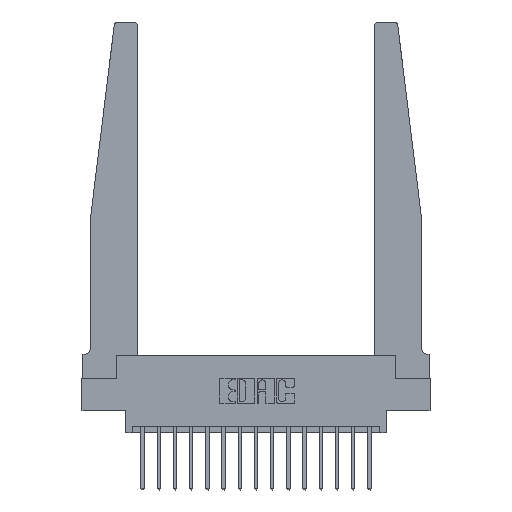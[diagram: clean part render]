
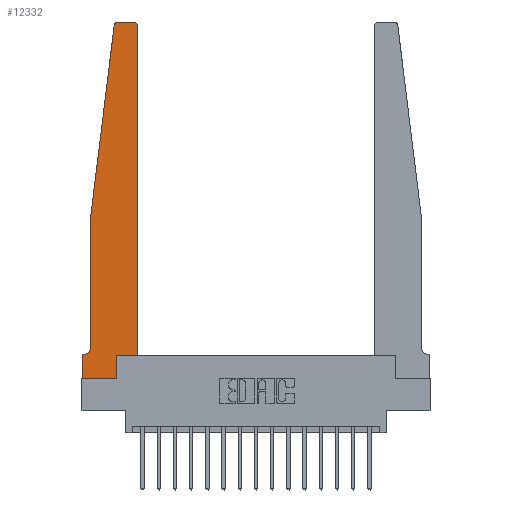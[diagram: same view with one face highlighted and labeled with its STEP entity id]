
A CAD part, top view. The second image highlights one B-rep face of the part: STEP entity #12332.
In plain terms, the highlighted planar face has unit normal (0, 0, 1).
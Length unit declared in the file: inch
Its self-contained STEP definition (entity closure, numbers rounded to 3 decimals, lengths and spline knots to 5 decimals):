
#579 = EDGE_CURVE ( 'NONE', #6346, #10243, #11988, .T. ) ;
#762 = CARTESIAN_POINT ( 'NONE',  ( 0.25, 2.75, 0.37 ) ) ;
#794 = CARTESIAN_POINT ( 'NONE',  ( 0., 0., 0.37 ) ) ;
#823 = DIRECTION ( 'NONE',  ( 0., 1., 0. ) ) ;
#884 = CARTESIAN_POINT ( 'NONE',  ( 0.2605, 0.18, 0.37 ) ) ;
#886 = VERTEX_POINT ( 'NONE', #3047 ) ;
#998 = AXIS2_PLACEMENT_3D ( 'NONE', #14001, #2304, #3636 ) ;
#999 = ORIENTED_EDGE ( 'NONE', *, *, #14051, .T. ) ;
#1044 = VECTOR ( 'NONE', #5121, 39.37008 ) ;
#1132 = DIRECTION ( 'NONE',  ( 1., 0., 0. ) ) ;
#1226 = CARTESIAN_POINT ( 'NONE',  ( 0.27653, 2.72, 0.37 ) ) ;
#1309 = EDGE_CURVE ( 'NONE', #12585, #11449, #10098, .T. ) ;
#1338 = DIRECTION ( 'NONE',  ( 0., -1., 0. ) ) ;
#2133 = CARTESIAN_POINT ( 'NONE',  ( 0.425, 0.18, 0.37 ) ) ;
#2304 = DIRECTION ( 'NONE',  ( 0., 0., -1. ) ) ;
#2358 = LINE ( 'NONE', #5302, #14975 ) ;
#2757 = LINE ( 'NONE', #8523, #7463 ) ;
#2759 = EDGE_LOOP ( 'NONE', ( #15138, #10796, #14246, #8769, #17786, #15051, #4332, #9977, #999, #9576, #3891, #8367 ) ) ;
#2890 = CARTESIAN_POINT ( 'NONE',  ( 0.395, 2.75, 0.37 ) ) ;
#3002 = EDGE_CURVE ( 'NONE', #10470, #3756, #13809, .T. ) ;
#3032 = DIRECTION ( 'NONE',  ( 0., 0., 1. ) ) ;
#3047 = CARTESIAN_POINT ( 'NONE',  ( 0.015, 0.1875, 0.37 ) ) ;
#3440 = EDGE_CURVE ( 'NONE', #886, #18617, #17401, .T. ) ;
#3474 = EDGE_CURVE ( 'NONE', #10243, #5282, #6529, .T. ) ;
#3499 = DIRECTION ( 'NONE',  ( 1., 0., 0. ) ) ;
#3636 = DIRECTION ( 'NONE',  ( -1., 0., 0. ) ) ;
#3689 = VECTOR ( 'NONE', #823, 39.37008 ) ;
#3756 = VERTEX_POINT ( 'NONE', #5103 ) ;
#3891 = ORIENTED_EDGE ( 'NONE', *, *, #579, .T. ) ;
#3909 = DIRECTION ( 'NONE',  ( 1., 0., 0. ) ) ;
#4058 = FACE_OUTER_BOUND ( 'NONE', #2759, .T. ) ;
#4332 = ORIENTED_EDGE ( 'NONE', *, *, #17624, .T. ) ;
#4445 = VERTEX_POINT ( 'NONE', #7677 ) ;
#4623 = EDGE_CURVE ( 'NONE', #11449, #4445, #2757, .T. ) ;
#4904 = CARTESIAN_POINT ( 'NONE',  ( 0.24675, 2.72367, 0.37 ) ) ;
#4949 = DIRECTION ( 'NONE',  ( 0., 1., 0. ) ) ;
#5032 = VECTOR ( 'NONE', #17313, 39.37008 ) ;
#5103 = CARTESIAN_POINT ( 'NONE',  ( 0.2605, 0., 0.37 ) ) ;
#5121 = DIRECTION ( 'NONE',  ( 0., -1., 0. ) ) ;
#5192 = VECTOR ( 'NONE', #4949, 39.37008 ) ;
#5282 = VERTEX_POINT ( 'NONE', #2890 ) ;
#5302 = CARTESIAN_POINT ( 'NONE',  ( 0.425, 0.18, 0.37 ) ) ;
#5584 = VERTEX_POINT ( 'NONE', #884 ) ;
#6346 = VERTEX_POINT ( 'NONE', #2133 ) ;
#6529 = CIRCLE ( 'NONE', #12309, 0.03 ) ;
#6906 = DIRECTION ( 'NONE',  ( 1., 0., 0. ) ) ;
#7148 = CARTESIAN_POINT ( 'NONE',  ( 0.065, 1.25, 0.37 ) ) ;
#7189 = VECTOR ( 'NONE', #11428, 39.37008 ) ;
#7250 = VERTEX_POINT ( 'NONE', #10916 ) ;
#7278 = CARTESIAN_POINT ( 'NONE',  ( 0.395, 2.72, 0.37 ) ) ;
#7463 = VECTOR ( 'NONE', #1338, 39.37008 ) ;
#7677 = CARTESIAN_POINT ( 'NONE',  ( 0.065, 0.2375, 0.37 ) ) ;
#8146 = CARTESIAN_POINT ( 'NONE',  ( 0., 0., 0.37 ) ) ;
#8236 = VECTOR ( 'NONE', #18435, 39.37008 ) ;
#8367 = ORIENTED_EDGE ( 'NONE', *, *, #3474, .T. ) ;
#8423 = LINE ( 'NONE', #11281, #1044 ) ;
#8523 = CARTESIAN_POINT ( 'NONE',  ( 0.065, 1.25, 0.37 ) ) ;
#8769 = ORIENTED_EDGE ( 'NONE', *, *, #4623, .T. ) ;
#9576 = ORIENTED_EDGE ( 'NONE', *, *, #15446, .T. ) ;
#9668 = DIRECTION ( 'NONE',  ( 0., 0., 1. ) ) ;
#9977 = ORIENTED_EDGE ( 'NONE', *, *, #3002, .T. ) ;
#10098 = LINE ( 'NONE', #7148, #7189 ) ;
#10243 = VERTEX_POINT ( 'NONE', #12563 ) ;
#10470 = VERTEX_POINT ( 'NONE', #8146 ) ;
#10796 = ORIENTED_EDGE ( 'NONE', *, *, #11027, .T. ) ;
#10916 = CARTESIAN_POINT ( 'NONE',  ( 0.27653, 2.75, 0.37 ) ) ;
#11027 = EDGE_CURVE ( 'NONE', #7250, #12585, #16127, .T. ) ;
#11281 = CARTESIAN_POINT ( 'NONE',  ( 0., 0., 0.37 ) ) ;
#11428 = DIRECTION ( 'NONE',  ( -0.122, -0.992, 0. ) ) ;
#11449 = VERTEX_POINT ( 'NONE', #15720 ) ;
#11465 = DIRECTION ( 'NONE',  ( 1., 0., 0. ) ) ;
#11988 = LINE ( 'NONE', #13694, #5192 ) ;
#12309 = AXIS2_PLACEMENT_3D ( 'NONE', #7278, #3032, #6906 ) ;
#12332 = ADVANCED_FACE ( 'NONE', ( #4058 ), #18428, .T. ) ;
#12563 = CARTESIAN_POINT ( 'NONE',  ( 0.425, 2.72, 0.37 ) ) ;
#12583 = LINE ( 'NONE', #12679, #3689 ) ;
#12585 = VERTEX_POINT ( 'NONE', #4904 ) ;
#12679 = CARTESIAN_POINT ( 'NONE',  ( 0.2605, 0.18, 0.37 ) ) ;
#12910 = VECTOR ( 'NONE', #3909, 39.37008 ) ;
#12961 = EDGE_CURVE ( 'NONE', #4445, #886, #13742, .T. ) ;
#13694 = CARTESIAN_POINT ( 'NONE',  ( 0.425, 0.18, 0.37 ) ) ;
#13742 = CIRCLE ( 'NONE', #998, 0.05 ) ;
#13809 = LINE ( 'NONE', #794, #12910 ) ;
#14001 = CARTESIAN_POINT ( 'NONE',  ( 0.015, 0.2375, 0.37 ) ) ;
#14051 = EDGE_CURVE ( 'NONE', #3756, #5584, #12583, .T. ) ;
#14246 = ORIENTED_EDGE ( 'NONE', *, *, #1309, .T. ) ;
#14448 = CARTESIAN_POINT ( 'NONE',  ( 0.065, 0.1875, 0.37 ) ) ;
#14612 = AXIS2_PLACEMENT_3D ( 'NONE', #1226, #9668, #11465 ) ;
#14928 = AXIS2_PLACEMENT_3D ( 'NONE', #15770, #18616, #1132 ) ;
#14975 = VECTOR ( 'NONE', #3499, 39.37008 ) ;
#15051 = ORIENTED_EDGE ( 'NONE', *, *, #3440, .T. ) ;
#15138 = ORIENTED_EDGE ( 'NONE', *, *, #17648, .T. ) ;
#15446 = EDGE_CURVE ( 'NONE', #5584, #6346, #2358, .T. ) ;
#15720 = CARTESIAN_POINT ( 'NONE',  ( 0.065, 1.25, 0.37 ) ) ;
#15770 = CARTESIAN_POINT ( 'NONE',  ( 0., 0.1875, 0.37 ) ) ;
#16127 = CIRCLE ( 'NONE', #14612, 0.03 ) ;
#16549 = CARTESIAN_POINT ( 'NONE',  ( 0., 0.1875, 0.37 ) ) ;
#17313 = DIRECTION ( 'NONE',  ( -1., 0., 0. ) ) ;
#17401 = LINE ( 'NONE', #14448, #5032 ) ;
#17624 = EDGE_CURVE ( 'NONE', #18617, #10470, #8423, .T. ) ;
#17648 = EDGE_CURVE ( 'NONE', #5282, #7250, #18253, .T. ) ;
#17786 = ORIENTED_EDGE ( 'NONE', *, *, #12961, .T. ) ;
#18253 = LINE ( 'NONE', #762, #8236 ) ;
#18428 = PLANE ( 'NONE',  #14928 ) ;
#18435 = DIRECTION ( 'NONE',  ( -1., 0., 0. ) ) ;
#18616 = DIRECTION ( 'NONE',  ( 0., 0., 1. ) ) ;
#18617 = VERTEX_POINT ( 'NONE', #16549 ) ;
